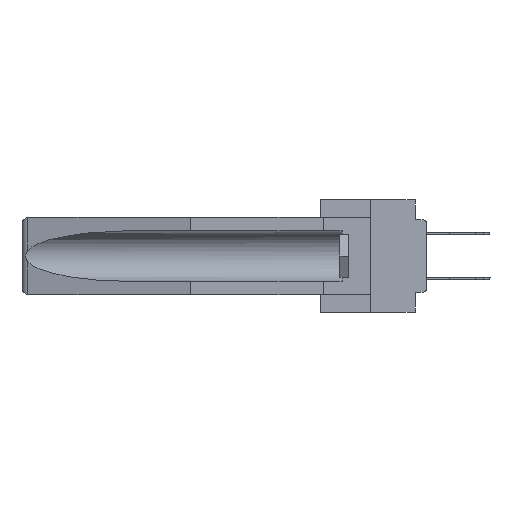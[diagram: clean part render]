
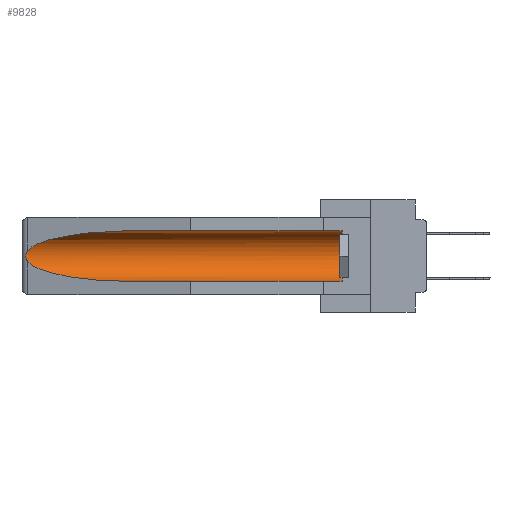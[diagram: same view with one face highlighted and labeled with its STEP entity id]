
A CAD part, left-side view. The second image highlights one B-rep face of the part: STEP entity #9828.
In plain terms, the highlighted cylindrical face has radius 2.857 mm (diameter 5.715 mm), a partial arc.
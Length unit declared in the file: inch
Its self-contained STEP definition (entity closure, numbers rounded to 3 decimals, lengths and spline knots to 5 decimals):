
#1371 = CARTESIAN_POINT ( 'NONE',  ( 0.26537, 1.52718, -0.19328 ) ) ;
#2336 = CARTESIAN_POINT ( 'NONE',  ( 0.25451, 1.48313, -0.09465 ) ) ;
#2836 = CARTESIAN_POINT ( 'NONE',  ( 0.2673, 1.53269, -0.17917 ) ) ;
#2860 = VERTEX_POINT ( 'NONE', #38070 ) ;
#5500 = CARTESIAN_POINT ( 'NONE',  ( 0.155, 1.07973, -0.059 ) ) ;
#6645 = EDGE_CURVE ( 'NONE', #33245, #26351, #9899, .T. ) ;
#6742 = ORIENTED_EDGE ( 'NONE', *, *, #37737, .T. ) ;
#6861 = CARTESIAN_POINT ( 'NONE',  ( 0.155, 0.126, -0.1715 ) ) ;
#7283 = EDGE_LOOP ( 'NONE', ( #30692, #6742, #14341, #24958, #16549, #34923 ) ) ;
#8293 = CIRCLE ( 'NONE', #38506, 0.1125 ) ;
#8510 = CARTESIAN_POINT ( 'NONE',  ( 0.2675, 1.53308, -0.16763 ) ) ;
#8774 = CARTESIAN_POINT ( 'NONE',  ( 0.26654, 1.53092, -0.15636 ) ) ;
#9048 =( BOUNDED_CURVE ( )  B_SPLINE_CURVE ( 3, ( #5500, #38416, #2336, #26334 ),
 .UNSPECIFIED., .F., .F. ) 
 B_SPLINE_CURVE_WITH_KNOTS ( ( 4, 4 ),
 ( 4.71239, 6.08839 ),
 .UNSPECIFIED. ) 
 CURVE ( )  GEOMETRIC_REPRESENTATION_ITEM ( )  RATIONAL_B_SPLINE_CURVE ( ( 1., 0.848, 0.848, 1. ) ) 
 REPRESENTATION_ITEM ( '' )  );
#9651 = EDGE_CURVE ( 'NONE', #20608, #33676, #35400, .T. ) ;
#9828 = ADVANCED_FACE ( 'NONE', ( #22670 ), #21194, .F. ) ;
#9891 = DIRECTION ( 'NONE',  ( 0., 0., 1. ) ) ;
#9899 = LINE ( 'NONE', #23288, #21686 ) ;
#10138 = DIRECTION ( 'NONE',  ( 0., 1., 0. ) ) ;
#12794 = EDGE_CURVE ( 'NONE', #32666, #33245, #8293, .T. ) ;
#13789 = CARTESIAN_POINT ( 'NONE',  ( 0.155, 0.126, -0.059 ) ) ;
#14341 = ORIENTED_EDGE ( 'NONE', *, *, #9651, .T. ) ;
#14581 = CARTESIAN_POINT ( 'NONE',  ( 0.26597, 1.52961, -0.15275 ) ) ;
#15226 = CARTESIAN_POINT ( 'NONE',  ( 0.26537, 1.52718, -0.19328 ) ) ;
#16549 = ORIENTED_EDGE ( 'NONE', *, *, #12794, .T. ) ;
#17201 = EDGE_CURVE ( 'NONE', #26351, #2860, #9048, .T. ) ;
#17344 = DIRECTION ( 'NONE',  ( 0., 0., 1. ) ) ;
#17865 = CARTESIAN_POINT ( 'NONE',  ( 0.26537, 1.52718, -0.14972 ) ) ;
#19587 = CARTESIAN_POINT ( 'NONE',  ( 0.155, 1.07973, -0.284 ) ) ;
#20608 = VERTEX_POINT ( 'NONE', #1371 ) ;
#20886 = CARTESIAN_POINT ( 'NONE',  ( 0.2673, 1.5327, -0.16383 ) ) ;
#21194 = CYLINDRICAL_SURFACE ( 'NONE', #31364, 0.1125 ) ;
#21389 = CARTESIAN_POINT ( 'NONE',  ( 0.155, 1.07973, -0.284 ) ) ;
#21686 = VECTOR ( 'NONE', #26425, 39.37008 ) ;
#22154 = CARTESIAN_POINT ( 'NONE',  ( 0.155, 1.07973, -0.059 ) ) ;
#22510 = CARTESIAN_POINT ( 'NONE',  ( 0.26537, 1.52718, -0.19328 ) ) ;
#22670 = FACE_OUTER_BOUND ( 'NONE', #7283, .T. ) ;
#22908 = CARTESIAN_POINT ( 'NONE',  ( 0.25451, 1.48313, -0.24835 ) ) ;
#23288 = CARTESIAN_POINT ( 'NONE',  ( 0.155, -0.30754, -0.059 ) ) ;
#23666 = DIRECTION ( 'NONE',  ( 0., 1., 0. ) ) ;
#24958 = ORIENTED_EDGE ( 'NONE', *, *, #32485, .F. ) ;
#26334 = CARTESIAN_POINT ( 'NONE',  ( 0.26537, 1.52718, -0.14972 ) ) ;
#26351 = VERTEX_POINT ( 'NONE', #22154 ) ;
#26425 = DIRECTION ( 'NONE',  ( 0., 1., 0. ) ) ;
#27932 = DIRECTION ( 'NONE',  ( 0., -1., 0. ) ) ;
#28585 = CARTESIAN_POINT ( 'NONE',  ( 0.155, -0.30754, -0.284 ) ) ;
#29572 = CARTESIAN_POINT ( 'NONE',  ( 0.2675, 1.53308, -0.17534 ) ) ;
#30050 = LINE ( 'NONE', #28585, #35222 ) ;
#30445 = CARTESIAN_POINT ( 'NONE',  ( 0.26655, 1.53094, -0.18657 ) ) ;
#30692 = ORIENTED_EDGE ( 'NONE', *, *, #17201, .T. ) ;
#31364 = AXIS2_PLACEMENT_3D ( 'NONE', #35610, #23666, #17344 ) ;
#32485 = EDGE_CURVE ( 'NONE', #32666, #33676, #30050, .T. ) ;
#32666 = VERTEX_POINT ( 'NONE', #38287 ) ;
#32937 = B_SPLINE_CURVE_WITH_KNOTS ( 'NONE', 3,
 ( #17865, #14581, #8774, #20886, #8510, #29572, #2836, #30445, #33346, #15226 ),
 .UNSPECIFIED., .F., .F.,
 ( 4, 2, 2, 2, 4 ),
 ( 0., 0.00029, 0.00058, 0.00087, 0.00117 ),
 .UNSPECIFIED. ) ;
#33245 = VERTEX_POINT ( 'NONE', #13789 ) ;
#33346 = CARTESIAN_POINT ( 'NONE',  ( 0.26597, 1.5296, -0.19026 ) ) ;
#33676 = VERTEX_POINT ( 'NONE', #21389 ) ;
#34582 = CARTESIAN_POINT ( 'NONE',  ( 0.21114, 1.30732, -0.284 ) ) ;
#34923 = ORIENTED_EDGE ( 'NONE', *, *, #6645, .T. ) ;
#35222 = VECTOR ( 'NONE', #10138, 39.37008 ) ;
#35400 =( BOUNDED_CURVE ( )  B_SPLINE_CURVE ( 3, ( #22510, #22908, #34582, #19587 ),
 .UNSPECIFIED., .F., .F. ) 
 B_SPLINE_CURVE_WITH_KNOTS ( ( 4, 4 ),
 ( 0.1948, 1.5708 ),
 .UNSPECIFIED. ) 
 CURVE ( )  GEOMETRIC_REPRESENTATION_ITEM ( )  RATIONAL_B_SPLINE_CURVE ( ( 1., 0.848, 0.848, 1. ) ) 
 REPRESENTATION_ITEM ( '' )  );
#35610 = CARTESIAN_POINT ( 'NONE',  ( 0.155, -0.30754, -0.1715 ) ) ;
#37737 = EDGE_CURVE ( 'NONE', #2860, #20608, #32937, .T. ) ;
#38070 = CARTESIAN_POINT ( 'NONE',  ( 0.26537, 1.52718, -0.14972 ) ) ;
#38287 = CARTESIAN_POINT ( 'NONE',  ( 0.155, 0.126, -0.284 ) ) ;
#38416 = CARTESIAN_POINT ( 'NONE',  ( 0.21114, 1.30732, -0.059 ) ) ;
#38506 = AXIS2_PLACEMENT_3D ( 'NONE', #6861, #27932, #9891 ) ;
